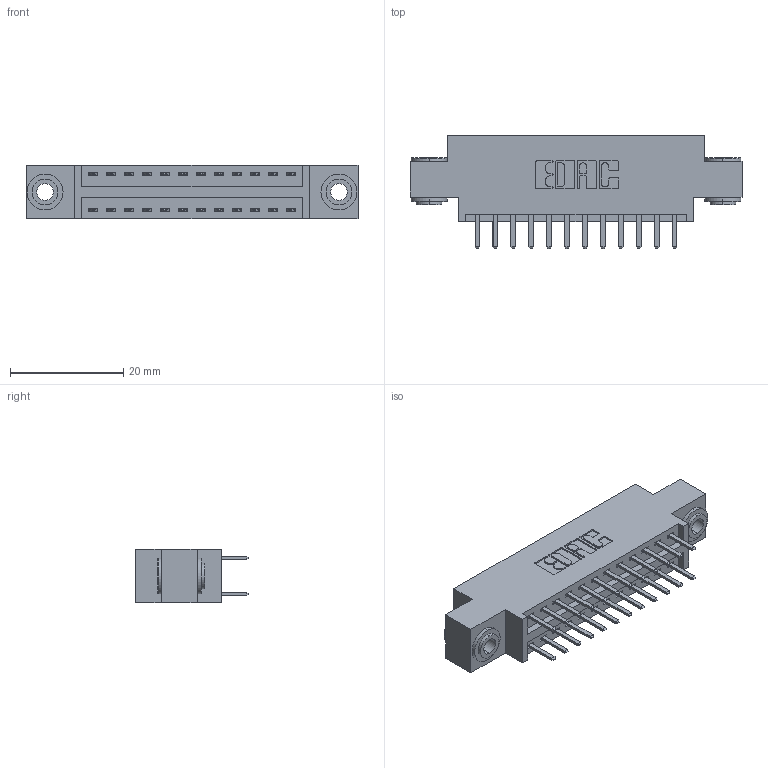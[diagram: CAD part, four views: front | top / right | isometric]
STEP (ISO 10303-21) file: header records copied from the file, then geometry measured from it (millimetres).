
FILE_DESCRIPTION (( 'STEP AP203' ), '1' );
FILE_NAME ('346-024-520-803.STEP', '2022-05-18T22:48:14', ( '' ), ( '' ), 'SwSTEP 2.0', 'SolidWorks 2020', '' );
FILE_SCHEMA (( 'CONFIG_CONTROL_DESIGN' ));
Length unit declared in the file: inch
Products named in the file (4): 345-292-001_345-293-120; 345-250-002_345-250-002-102; 346-024-520-803; 346 Part_0.170 Offset - 0.156 Dia-TH
Assembly tree (27 placements, depth 2):
  346-024-520-803
    346 Part_0.170 Offset - 0.156 Dia-TH
    345-292-001_345-293-120  x24
    345-250-002_345-250-002-102  x2
Bounding box: 58.67 x 20.02 x 9.4 mm (x, y, z)
Volume: 5324.6 mm3; surface area: 7251.1 mm2
Topology: 27 solids, 27 shells, 1522 faces, 4365 edges, 2842 vertices
Faces by surface type: plane 992, cylinder 522, cone 8
Entity records: 13182 total; most frequent: CARTESIAN_POINT 2209, ORIENTED_EDGE 2122, DIRECTION 2015, EDGE_CURVE 1061, VECTOR 853, LINE 853, VERTEX_POINT 702, AXIS2_PLACEMENT_3D 581
